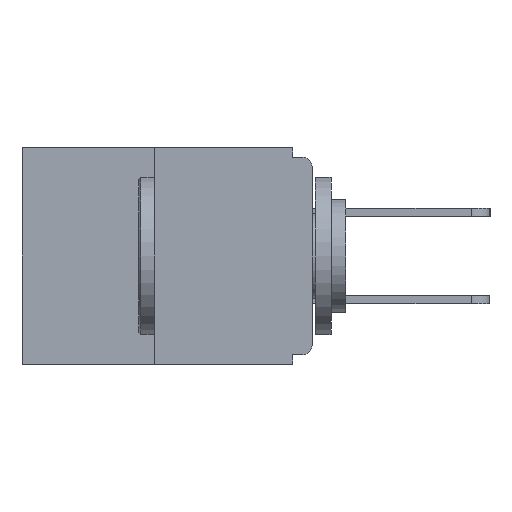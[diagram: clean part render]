
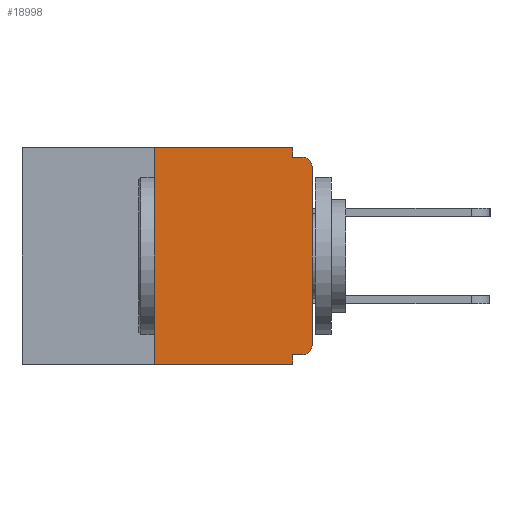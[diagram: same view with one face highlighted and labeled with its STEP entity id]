
A CAD part, left-side view. The second image highlights one B-rep face of the part: STEP entity #18998.
In plain terms, the highlighted planar face has unit normal (-1, 0, 0).
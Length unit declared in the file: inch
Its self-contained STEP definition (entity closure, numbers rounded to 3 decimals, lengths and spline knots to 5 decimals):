
#71 = CARTESIAN_POINT ( 'NONE',  ( 0., 0.031, -0.328 ) ) ;
#107 = EDGE_CURVE ( 'NONE', #18675, #12134, #23264, .T. ) ;
#112 = AXIS2_PLACEMENT_3D ( 'NONE', #4386, #17038, #22231 ) ;
#264 = LINE ( 'NONE', #15448, #4817 ) ;
#1315 = ORIENTED_EDGE ( 'NONE', *, *, #7322, .F. ) ;
#1703 = AXIS2_PLACEMENT_3D ( 'NONE', #14887, #16740, #5987 ) ;
#2218 = VERTEX_POINT ( 'NONE', #2459 ) ;
#2223 = ORIENTED_EDGE ( 'NONE', *, *, #14469, .T. ) ;
#2459 = CARTESIAN_POINT ( 'NONE',  ( 0., 0., -0.313 ) ) ;
#2510 = VERTEX_POINT ( 'NONE', #71 ) ;
#3694 = CARTESIAN_POINT ( 'NONE',  ( 0., 0., 0. ) ) ;
#4132 = ORIENTED_EDGE ( 'NONE', *, *, #17138, .F. ) ;
#4317 = VERTEX_POINT ( 'NONE', #23071 ) ;
#4386 = CARTESIAN_POINT ( 'NONE',  ( 0., 0.015, -0.03 ) ) ;
#4817 = VECTOR ( 'NONE', #17465, 39.37008 ) ;
#4959 = ORIENTED_EDGE ( 'NONE', *, *, #7828, .F. ) ;
#5289 = PLANE ( 'NONE',  #16008 ) ;
#5341 = EDGE_LOOP ( 'NONE', ( #12326, #4959, #2223, #4132, #10049, #6519, #18918, #19238, #12515, #1315 ) ) ;
#5701 = VERTEX_POINT ( 'NONE', #14086 ) ;
#5895 = FACE_OUTER_BOUND ( 'NONE', #5341, .T. ) ;
#5987 = DIRECTION ( 'NONE',  ( 0., 0., -1. ) ) ;
#6519 = ORIENTED_EDGE ( 'NONE', *, *, #11186, .T. ) ;
#6543 = CARTESIAN_POINT ( 'NONE',  ( 0., 0.031, 0. ) ) ;
#7101 = VECTOR ( 'NONE', #22270, 39.37008 ) ;
#7322 = EDGE_CURVE ( 'NONE', #12134, #5701, #11868, .T. ) ;
#7521 = LINE ( 'NONE', #10921, #17964 ) ;
#7775 = CIRCLE ( 'NONE', #1703, 0.015 ) ;
#7828 = EDGE_CURVE ( 'NONE', #4317, #18675, #18095, .T. ) ;
#8493 = DIRECTION ( 'NONE',  ( 0., -1., 0. ) ) ;
#8986 = DIRECTION ( 'NONE',  ( 1., 0., 0. ) ) ;
#9165 = CARTESIAN_POINT ( 'NONE',  ( 0., 0., -0.015 ) ) ;
#9298 = VECTOR ( 'NONE', #19827, 39.37008 ) ;
#9485 = VECTOR ( 'NONE', #12314, 39.37008 ) ;
#9952 = CARTESIAN_POINT ( 'NONE',  ( 0., 0.46, 0. ) ) ;
#9965 = CARTESIAN_POINT ( 'NONE',  ( 0., 0.015, -0.015 ) ) ;
#10049 = ORIENTED_EDGE ( 'NONE', *, *, #20680, .F. ) ;
#10614 = CARTESIAN_POINT ( 'NONE',  ( 0., 0.031, -0.343 ) ) ;
#10801 = DIRECTION ( 'NONE',  ( 0., 0., -1. ) ) ;
#10921 = CARTESIAN_POINT ( 'NONE',  ( 0., 0., -0.328 ) ) ;
#10972 = DIRECTION ( 'NONE',  ( 0., -1., 0. ) ) ;
#11186 = EDGE_CURVE ( 'NONE', #14509, #2218, #7775, .T. ) ;
#11311 = VECTOR ( 'NONE', #8493, 39.37008 ) ;
#11591 = CARTESIAN_POINT ( 'NONE',  ( 0., 0.25, 0. ) ) ;
#11868 = LINE ( 'NONE', #20204, #7101 ) ;
#12134 = VERTEX_POINT ( 'NONE', #6543 ) ;
#12314 = DIRECTION ( 'NONE',  ( 0., -1., 0. ) ) ;
#12326 = ORIENTED_EDGE ( 'NONE', *, *, #107, .F. ) ;
#12474 = DIRECTION ( 'NONE',  ( 0., 1., 0. ) ) ;
#12515 = ORIENTED_EDGE ( 'NONE', *, *, #20886, .F. ) ;
#12687 = CARTESIAN_POINT ( 'NONE',  ( 0., 0.46, 0. ) ) ;
#14086 = CARTESIAN_POINT ( 'NONE',  ( 0., 0.031, -0.015 ) ) ;
#14469 = EDGE_CURVE ( 'NONE', #4317, #16958, #19084, .T. ) ;
#14509 = VERTEX_POINT ( 'NONE', #16073 ) ;
#14887 = CARTESIAN_POINT ( 'NONE',  ( 0., 0.015, -0.313 ) ) ;
#15233 = CARTESIAN_POINT ( 'NONE',  ( 0., 0.46, -0.343 ) ) ;
#15448 = CARTESIAN_POINT ( 'NONE',  ( 0., 0.031, -0.343 ) ) ;
#15683 = LINE ( 'NONE', #9165, #22526 ) ;
#16008 = AXIS2_PLACEMENT_3D ( 'NONE', #12687, #8986, #10801 ) ;
#16073 = CARTESIAN_POINT ( 'NONE',  ( 0., 0.015, -0.328 ) ) ;
#16566 = VERTEX_POINT ( 'NONE', #22805 ) ;
#16740 = DIRECTION ( 'NONE',  ( -1., 0., 0. ) ) ;
#16958 = VERTEX_POINT ( 'NONE', #10614 ) ;
#17038 = DIRECTION ( 'NONE',  ( -1., 0., 0. ) ) ;
#17056 = CIRCLE ( 'NONE', #112, 0.015 ) ;
#17138 = EDGE_CURVE ( 'NONE', #2510, #16958, #264, .T. ) ;
#17465 = DIRECTION ( 'NONE',  ( 0., 0., -1. ) ) ;
#17696 = VERTEX_POINT ( 'NONE', #9965 ) ;
#17836 = EDGE_CURVE ( 'NONE', #2218, #16566, #20651, .T. ) ;
#17964 = VECTOR ( 'NONE', #12474, 39.37008 ) ;
#18095 = LINE ( 'NONE', #22251, #20097 ) ;
#18675 = VERTEX_POINT ( 'NONE', #11591 ) ;
#18918 = ORIENTED_EDGE ( 'NONE', *, *, #17836, .T. ) ;
#18998 = ADVANCED_FACE ( 'NONE', ( #5895 ), #5289, .F. ) ;
#19084 = LINE ( 'NONE', #15233, #9485 ) ;
#19238 = ORIENTED_EDGE ( 'NONE', *, *, #21778, .T. ) ;
#19827 = DIRECTION ( 'NONE',  ( 0., 0., 1. ) ) ;
#20097 = VECTOR ( 'NONE', #21957, 39.37008 ) ;
#20204 = CARTESIAN_POINT ( 'NONE',  ( 0., 0.031, 0. ) ) ;
#20651 = LINE ( 'NONE', #3694, #9298 ) ;
#20680 = EDGE_CURVE ( 'NONE', #14509, #2510, #7521, .T. ) ;
#20886 = EDGE_CURVE ( 'NONE', #5701, #17696, #15683, .T. ) ;
#21778 = EDGE_CURVE ( 'NONE', #16566, #17696, #17056, .T. ) ;
#21957 = DIRECTION ( 'NONE',  ( 0., 0., 1. ) ) ;
#22231 = DIRECTION ( 'NONE',  ( 0., 0., -1. ) ) ;
#22251 = CARTESIAN_POINT ( 'NONE',  ( 0., 0.25, 0. ) ) ;
#22270 = DIRECTION ( 'NONE',  ( 0., 0., -1. ) ) ;
#22526 = VECTOR ( 'NONE', #10972, 39.37008 ) ;
#22805 = CARTESIAN_POINT ( 'NONE',  ( 0., 0., -0.03 ) ) ;
#23071 = CARTESIAN_POINT ( 'NONE',  ( 0., 0.25, -0.343 ) ) ;
#23264 = LINE ( 'NONE', #9952, #11311 ) ;
